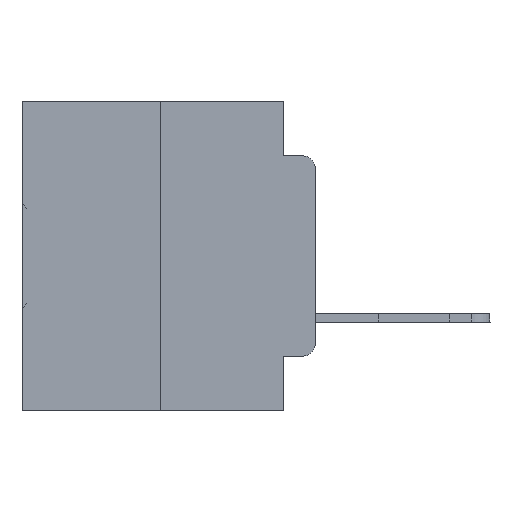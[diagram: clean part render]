
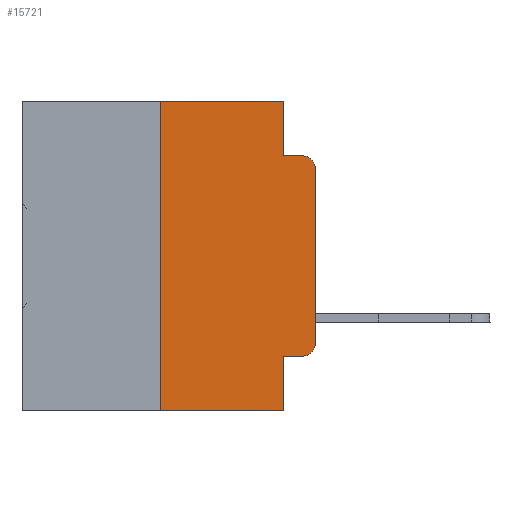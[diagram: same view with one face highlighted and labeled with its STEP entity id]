
A CAD part, left-side view. The second image highlights one B-rep face of the part: STEP entity #15721.
In plain terms, the highlighted planar face has unit normal (-1, 0, 0).
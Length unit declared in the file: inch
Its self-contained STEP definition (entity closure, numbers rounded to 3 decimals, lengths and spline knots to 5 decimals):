
#18 = EDGE_CURVE ( 'NONE', #15138, #29613, #20262, .T. ) ;
#120 = EDGE_CURVE ( 'NONE', #16273, #7164, #1326, .T. ) ;
#293 = CARTESIAN_POINT ( 'NONE',  ( 0., 0.473, -0.5 ) ) ;
#324 = CARTESIAN_POINT ( 'NONE',  ( 0., 0.25, 0. ) ) ;
#489 = ORIENTED_EDGE ( 'NONE', *, *, #23193, .F. ) ;
#931 = EDGE_LOOP ( 'NONE', ( #32824, #3843, #489, #23143, #21458, #6390, #26710, #31570, #31605, #3457 ) ) ;
#1070 = CIRCLE ( 'NONE', #1973, 0.02 ) ;
#1237 = VERTEX_POINT ( 'NONE', #15448 ) ;
#1326 = LINE ( 'NONE', #12139, #12181 ) ;
#1832 = DIRECTION ( 'NONE',  ( -1., 0., 0. ) ) ;
#1973 = AXIS2_PLACEMENT_3D ( 'NONE', #6633, #17732, #20508 ) ;
#2248 = CARTESIAN_POINT ( 'NONE',  ( 0., 0.25, 0. ) ) ;
#2455 = DIRECTION ( 'NONE',  ( 0., -1., 0. ) ) ;
#3449 = VERTEX_POINT ( 'NONE', #7341 ) ;
#3457 = ORIENTED_EDGE ( 'NONE', *, *, #28179, .T. ) ;
#3843 = ORIENTED_EDGE ( 'NONE', *, *, #30294, .T. ) ;
#5346 = CARTESIAN_POINT ( 'NONE',  ( 0., 0.051, 0. ) ) ;
#5658 = AXIS2_PLACEMENT_3D ( 'NONE', #11789, #29896, #14401 ) ;
#5660 = DIRECTION ( 'NONE',  ( 0., 0., 1. ) ) ;
#6193 = VECTOR ( 'NONE', #10920, 39.37008 ) ;
#6390 = ORIENTED_EDGE ( 'NONE', *, *, #24746, .F. ) ;
#6536 = DIRECTION ( 'NONE',  ( 0., -1., 0. ) ) ;
#6633 = CARTESIAN_POINT ( 'NONE',  ( 0., 0.02, -0.3915 ) ) ;
#7164 = VERTEX_POINT ( 'NONE', #11905 ) ;
#7341 = CARTESIAN_POINT ( 'NONE',  ( 0., 0.02, -0.0885 ) ) ;
#8214 = VERTEX_POINT ( 'NONE', #24164 ) ;
#8515 = VECTOR ( 'NONE', #5660, 39.37008 ) ;
#8855 = CARTESIAN_POINT ( 'NONE',  ( 0., 0.051, -0.0885 ) ) ;
#10240 = CARTESIAN_POINT ( 'NONE',  ( 0., 0.051, 0. ) ) ;
#10463 = DIRECTION ( 'NONE',  ( 0., 0., -1. ) ) ;
#10904 = VECTOR ( 'NONE', #2455, 39.37008 ) ;
#10920 = DIRECTION ( 'NONE',  ( 0., -1., 0. ) ) ;
#11789 = CARTESIAN_POINT ( 'NONE',  ( 0., 0.473, 0. ) ) ;
#11905 = CARTESIAN_POINT ( 'NONE',  ( 0., 0., -0.1085 ) ) ;
#11967 = VERTEX_POINT ( 'NONE', #12093 ) ;
#12093 = CARTESIAN_POINT ( 'NONE',  ( 0., 0.051, -0.4115 ) ) ;
#12139 = CARTESIAN_POINT ( 'NONE',  ( 0., 0., 0. ) ) ;
#12181 = VECTOR ( 'NONE', #32808, 39.37008 ) ;
#12312 = VECTOR ( 'NONE', #21920, 39.37008 ) ;
#13525 = CARTESIAN_POINT ( 'NONE',  ( 0., 0.02, -0.4115 ) ) ;
#13577 = LINE ( 'NONE', #8855, #12312 ) ;
#14401 = DIRECTION ( 'NONE',  ( 0., 0., -1. ) ) ;
#14683 = CARTESIAN_POINT ( 'NONE',  ( 0., 0.25, -0.5 ) ) ;
#15138 = VERTEX_POINT ( 'NONE', #2248 ) ;
#15448 = CARTESIAN_POINT ( 'NONE',  ( 0., 0.051, -0.0885 ) ) ;
#15721 = ADVANCED_FACE ( 'NONE', ( #25748 ), #24828, .F. ) ;
#15834 = DIRECTION ( 'NONE',  ( 0., 0., -1. ) ) ;
#15849 = EDGE_CURVE ( 'NONE', #29613, #1237, #23268, .T. ) ;
#16140 = CARTESIAN_POINT ( 'NONE',  ( 0., 0.473, 0. ) ) ;
#16273 = VERTEX_POINT ( 'NONE', #17588 ) ;
#17588 = CARTESIAN_POINT ( 'NONE',  ( 0., 0., -0.3915 ) ) ;
#17732 = DIRECTION ( 'NONE',  ( -1., 0., 0. ) ) ;
#18609 = LINE ( 'NONE', #293, #10904 ) ;
#20262 = LINE ( 'NONE', #16140, #6193 ) ;
#20472 = LINE ( 'NONE', #27319, #31440 ) ;
#20508 = DIRECTION ( 'NONE',  ( 0., 0., -1. ) ) ;
#20602 = CARTESIAN_POINT ( 'NONE',  ( 0., 0.051, 0. ) ) ;
#20755 = EDGE_CURVE ( 'NONE', #30862, #8214, #18609, .T. ) ;
#21458 = ORIENTED_EDGE ( 'NONE', *, *, #18, .F. ) ;
#21920 = DIRECTION ( 'NONE',  ( 0., -1., 0. ) ) ;
#23143 = ORIENTED_EDGE ( 'NONE', *, *, #15849, .F. ) ;
#23193 = EDGE_CURVE ( 'NONE', #1237, #3449, #13577, .T. ) ;
#23268 = LINE ( 'NONE', #5346, #29802 ) ;
#24164 = CARTESIAN_POINT ( 'NONE',  ( 0., 0.051, -0.5 ) ) ;
#24746 = EDGE_CURVE ( 'NONE', #30862, #15138, #25518, .T. ) ;
#24828 = PLANE ( 'NONE',  #5658 ) ;
#25432 = VECTOR ( 'NONE', #10463, 39.37008 ) ;
#25518 = LINE ( 'NONE', #324, #8515 ) ;
#25748 = FACE_OUTER_BOUND ( 'NONE', #931, .T. ) ;
#26279 = AXIS2_PLACEMENT_3D ( 'NONE', #30064, #1832, #30168 ) ;
#26420 = EDGE_CURVE ( 'NONE', #11967, #8214, #27469, .T. ) ;
#26710 = ORIENTED_EDGE ( 'NONE', *, *, #20755, .T. ) ;
#27179 = CIRCLE ( 'NONE', #26279, 0.02 ) ;
#27319 = CARTESIAN_POINT ( 'NONE',  ( 0., 0.051, -0.4115 ) ) ;
#27469 = LINE ( 'NONE', #20602, #25432 ) ;
#28179 = EDGE_CURVE ( 'NONE', #31637, #16273, #1070, .T. ) ;
#29613 = VERTEX_POINT ( 'NONE', #10240 ) ;
#29802 = VECTOR ( 'NONE', #15834, 39.37008 ) ;
#29896 = DIRECTION ( 'NONE',  ( 1., 0., 0. ) ) ;
#30064 = CARTESIAN_POINT ( 'NONE',  ( 0., 0.02, -0.1085 ) ) ;
#30168 = DIRECTION ( 'NONE',  ( 0., 0., -1. ) ) ;
#30294 = EDGE_CURVE ( 'NONE', #7164, #3449, #27179, .T. ) ;
#30862 = VERTEX_POINT ( 'NONE', #14683 ) ;
#31440 = VECTOR ( 'NONE', #6536, 39.37008 ) ;
#31570 = ORIENTED_EDGE ( 'NONE', *, *, #26420, .F. ) ;
#31605 = ORIENTED_EDGE ( 'NONE', *, *, #33094, .T. ) ;
#31637 = VERTEX_POINT ( 'NONE', #13525 ) ;
#32808 = DIRECTION ( 'NONE',  ( 0., 0., 1. ) ) ;
#32824 = ORIENTED_EDGE ( 'NONE', *, *, #120, .T. ) ;
#33094 = EDGE_CURVE ( 'NONE', #11967, #31637, #20472, .T. ) ;
